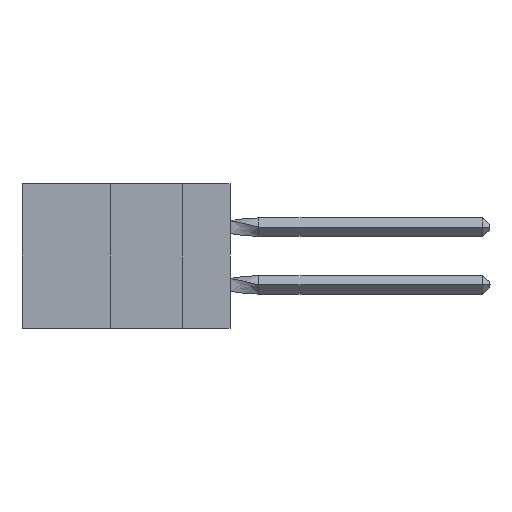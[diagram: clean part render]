
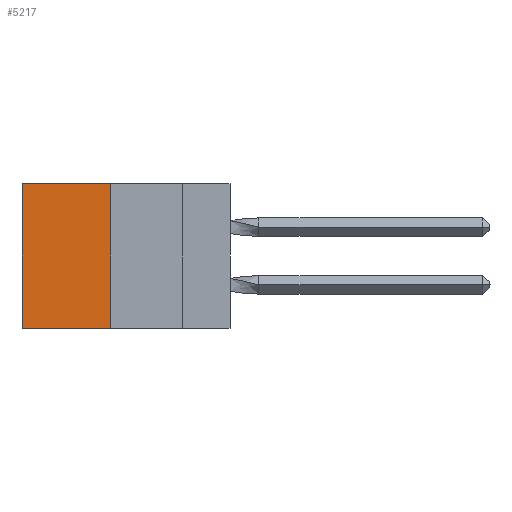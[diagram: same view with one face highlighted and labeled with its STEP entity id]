
A CAD part, left-side view. The second image highlights one B-rep face of the part: STEP entity #5217.
In plain terms, the highlighted planar face has unit normal (-1, 0, 0).
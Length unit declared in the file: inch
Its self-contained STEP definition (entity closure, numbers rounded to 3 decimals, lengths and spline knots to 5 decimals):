
#140 = VERTEX_POINT ( 'NONE', #13789 ) ;
#623 = DIRECTION ( 'NONE',  ( 0., 0., -1. ) ) ;
#979 = VERTEX_POINT ( 'NONE', #7459 ) ;
#1671 = ORIENTED_EDGE ( 'NONE', *, *, #7081, .T. ) ;
#1692 = CARTESIAN_POINT ( 'NONE',  ( 0.305, 0.72, -0.5 ) ) ;
#3310 = VERTEX_POINT ( 'NONE', #8056 ) ;
#3484 = EDGE_CURVE ( 'NONE', #979, #14855, #16459, .T. ) ;
#4400 = VECTOR ( 'NONE', #9865, 39.37008 ) ;
#5217 = ADVANCED_FACE ( 'NONE', ( #8484 ), #13280, .F. ) ;
#5496 = VECTOR ( 'NONE', #8633, 39.37008 ) ;
#5721 = ORIENTED_EDGE ( 'NONE', *, *, #3484, .T. ) ;
#6246 = ORIENTED_EDGE ( 'NONE', *, *, #9316, .F. ) ;
#6658 = CARTESIAN_POINT ( 'NONE',  ( 0.305, 0.413, -0.5 ) ) ;
#6921 = VECTOR ( 'NONE', #16826, 39.37008 ) ;
#7081 = EDGE_CURVE ( 'NONE', #14855, #3310, #17177, .T. ) ;
#7459 = CARTESIAN_POINT ( 'NONE',  ( 0.305, 0.413, 0. ) ) ;
#7926 = EDGE_CURVE ( 'NONE', #140, #3310, #10124, .T. ) ;
#8056 = CARTESIAN_POINT ( 'NONE',  ( 0.305, 0.72, -0.5 ) ) ;
#8374 = CARTESIAN_POINT ( 'NONE',  ( 0.305, 0.413, -0.5 ) ) ;
#8381 = DIRECTION ( 'NONE',  ( 1., 0., 0. ) ) ;
#8484 = FACE_OUTER_BOUND ( 'NONE', #14687, .T. ) ;
#8633 = DIRECTION ( 'NONE',  ( 0., 1., 0. ) ) ;
#9154 = VECTOR ( 'NONE', #623, 39.37008 ) ;
#9316 = EDGE_CURVE ( 'NONE', #979, #140, #14530, .T. ) ;
#9865 = DIRECTION ( 'NONE',  ( 0., 0., -1. ) ) ;
#10124 = LINE ( 'NONE', #11525, #6921 ) ;
#11525 = CARTESIAN_POINT ( 'NONE',  ( 0.305, 0.413, -0.5 ) ) ;
#12106 = CARTESIAN_POINT ( 'NONE',  ( 0.305, 0.72, 0. ) ) ;
#12125 = CARTESIAN_POINT ( 'NONE',  ( 0.305, 0.413, 0. ) ) ;
#13280 = PLANE ( 'NONE',  #15108 ) ;
#13789 = CARTESIAN_POINT ( 'NONE',  ( 0.305, 0.413, -0.5 ) ) ;
#13979 = ORIENTED_EDGE ( 'NONE', *, *, #7926, .F. ) ;
#14530 = LINE ( 'NONE', #8374, #4400 ) ;
#14687 = EDGE_LOOP ( 'NONE', ( #1671, #13979, #6246, #5721 ) ) ;
#14855 = VERTEX_POINT ( 'NONE', #12106 ) ;
#15061 = DIRECTION ( 'NONE',  ( 0., 0., -1. ) ) ;
#15108 = AXIS2_PLACEMENT_3D ( 'NONE', #6658, #8381, #15061 ) ;
#16459 = LINE ( 'NONE', #12125, #5496 ) ;
#16826 = DIRECTION ( 'NONE',  ( 0., 1., 0. ) ) ;
#17177 = LINE ( 'NONE', #1692, #9154 ) ;
